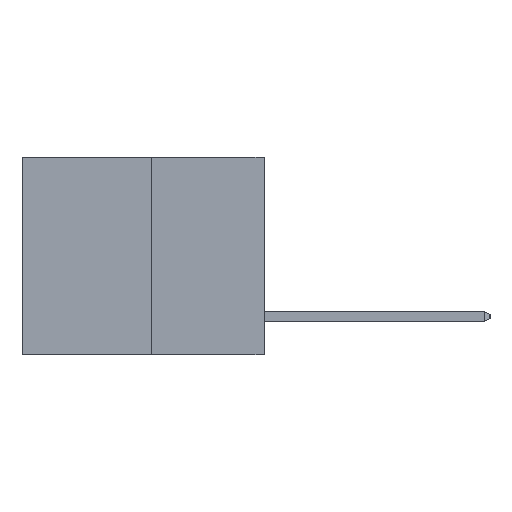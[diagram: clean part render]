
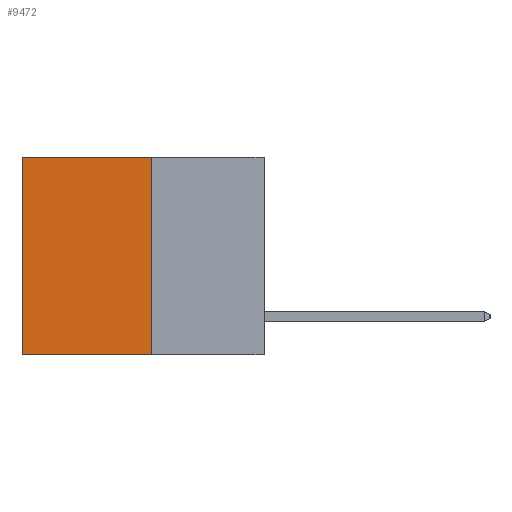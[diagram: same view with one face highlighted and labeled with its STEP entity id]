
A CAD part, left-side view. The second image highlights one B-rep face of the part: STEP entity #9472.
In plain terms, the highlighted planar face has unit normal (-1, 0, 0).
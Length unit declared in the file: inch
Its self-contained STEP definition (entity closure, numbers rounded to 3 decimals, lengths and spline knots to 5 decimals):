
#467 = ORIENTED_EDGE ( 'NONE', *, *, #1612, .F. ) ;
#492 = CARTESIAN_POINT ( 'NONE',  ( 0.3165, 0.28, -0.49 ) ) ;
#554 = DIRECTION ( 'NONE',  ( 0., 1., 0. ) ) ;
#1476 = LINE ( 'NONE', #1665, #7559 ) ;
#1612 = EDGE_CURVE ( 'NONE', #5346, #5779, #8824, .T. ) ;
#1665 = CARTESIAN_POINT ( 'NONE',  ( 0.3165, 0.28, -0.49 ) ) ;
#1736 = DIRECTION ( 'NONE',  ( 0., 1., 0. ) ) ;
#2034 = AXIS2_PLACEMENT_3D ( 'NONE', #492, #6189, #8042 ) ;
#3044 = DIRECTION ( 'NONE',  ( 0., 0., -1. ) ) ;
#3063 = VECTOR ( 'NONE', #554, 39.37008 ) ;
#3081 = CARTESIAN_POINT ( 'NONE',  ( 0.3165, 0.6, -0.49 ) ) ;
#3325 = VECTOR ( 'NONE', #1736, 39.37008 ) ;
#4215 = ORIENTED_EDGE ( 'NONE', *, *, #9781, .T. ) ;
#4557 = LINE ( 'NONE', #3081, #6786 ) ;
#4584 = CARTESIAN_POINT ( 'NONE',  ( 0.3165, 0.6, 0. ) ) ;
#4939 = CARTESIAN_POINT ( 'NONE',  ( 0.3165, 0.28, 0. ) ) ;
#5073 = EDGE_CURVE ( 'NONE', #7507, #5346, #1476, .T. ) ;
#5346 = VERTEX_POINT ( 'NONE', #6760 ) ;
#5779 = VERTEX_POINT ( 'NONE', #8455 ) ;
#6189 = DIRECTION ( 'NONE',  ( 1., 0., 0. ) ) ;
#6375 = VERTEX_POINT ( 'NONE', #4584 ) ;
#6760 = CARTESIAN_POINT ( 'NONE',  ( 0.3165, 0.28, -0.49 ) ) ;
#6786 = VECTOR ( 'NONE', #3044, 39.37008 ) ;
#7159 = CARTESIAN_POINT ( 'NONE',  ( 0.3165, 0.28, 0. ) ) ;
#7507 = VERTEX_POINT ( 'NONE', #4939 ) ;
#7559 = VECTOR ( 'NONE', #10089, 39.37008 ) ;
#7909 = ORIENTED_EDGE ( 'NONE', *, *, #9831, .T. ) ;
#8042 = DIRECTION ( 'NONE',  ( 0., 0., -1. ) ) ;
#8282 = CARTESIAN_POINT ( 'NONE',  ( 0.3165, 0.28, -0.49 ) ) ;
#8455 = CARTESIAN_POINT ( 'NONE',  ( 0.3165, 0.6, -0.49 ) ) ;
#8824 = LINE ( 'NONE', #8282, #3325 ) ;
#9003 = PLANE ( 'NONE',  #2034 ) ;
#9472 = ADVANCED_FACE ( 'NONE', ( #9885 ), #9003, .F. ) ;
#9781 = EDGE_CURVE ( 'NONE', #6375, #5779, #4557, .T. ) ;
#9831 = EDGE_CURVE ( 'NONE', #7507, #6375, #9874, .T. ) ;
#9874 = LINE ( 'NONE', #7159, #3063 ) ;
#9875 = ORIENTED_EDGE ( 'NONE', *, *, #5073, .F. ) ;
#9885 = FACE_OUTER_BOUND ( 'NONE', #11719, .T. ) ;
#10089 = DIRECTION ( 'NONE',  ( 0., 0., -1. ) ) ;
#11719 = EDGE_LOOP ( 'NONE', ( #4215, #467, #9875, #7909 ) ) ;
